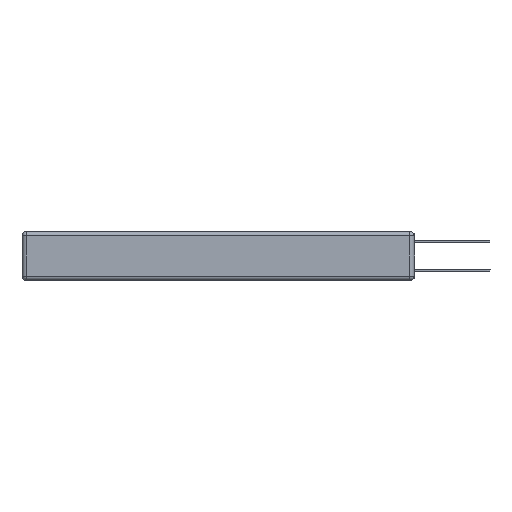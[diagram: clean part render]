
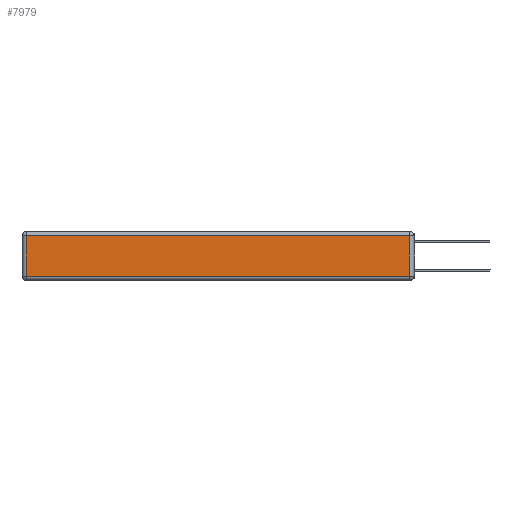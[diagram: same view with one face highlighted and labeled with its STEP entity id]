
A CAD part, left-side view. The second image highlights one B-rep face of the part: STEP entity #7979.
In plain terms, the highlighted planar face has unit normal (-1, 0, 0).
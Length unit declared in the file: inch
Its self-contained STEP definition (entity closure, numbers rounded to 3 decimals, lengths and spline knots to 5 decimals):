
#330 = VECTOR ( 'NONE', #3692, 39.37008 ) ;
#1174 = CARTESIAN_POINT ( 'NONE',  ( 0., 2.72, -0.343 ) ) ;
#1606 = ORIENTED_EDGE ( 'NONE', *, *, #9624, .T. ) ;
#1670 = VERTEX_POINT ( 'NONE', #16334 ) ;
#1967 = CARTESIAN_POINT ( 'NONE',  ( 0., 2.75, -0.03 ) ) ;
#2464 = EDGE_CURVE ( 'NONE', #16041, #1670, #11679, .T. ) ;
#2591 = DIRECTION ( 'NONE',  ( 0., 0., 1. ) ) ;
#3074 = CARTESIAN_POINT ( 'NONE',  ( 0., 0., -0.343 ) ) ;
#3692 = DIRECTION ( 'NONE',  ( 0., 0., -1. ) ) ;
#3740 = CARTESIAN_POINT ( 'NONE',  ( 0., 0.03, -0.313 ) ) ;
#4265 = LINE ( 'NONE', #9341, #16293 ) ;
#4415 = PLANE ( 'NONE',  #5699 ) ;
#5323 = VECTOR ( 'NONE', #11095, 39.37008 ) ;
#5699 = AXIS2_PLACEMENT_3D ( 'NONE', #3074, #6194, #8405 ) ;
#6194 = DIRECTION ( 'NONE',  ( -1., 0., 0. ) ) ;
#6601 = FACE_OUTER_BOUND ( 'NONE', #9531, .T. ) ;
#6953 = LINE ( 'NONE', #8497, #5323 ) ;
#7979 = ADVANCED_FACE ( 'NONE', ( #6601 ), #4415, .T. ) ;
#8330 = CARTESIAN_POINT ( 'NONE',  ( 0., 2.72, -0.03 ) ) ;
#8405 = DIRECTION ( 'NONE',  ( 0., 0., 1. ) ) ;
#8497 = CARTESIAN_POINT ( 'NONE',  ( 0., 0., -0.313 ) ) ;
#9250 = EDGE_CURVE ( 'NONE', #1670, #14311, #6953, .T. ) ;
#9341 = CARTESIAN_POINT ( 'NONE',  ( 0., 0.03, -0.343 ) ) ;
#9531 = EDGE_LOOP ( 'NONE', ( #9869, #1606, #12009, #12300 ) ) ;
#9624 = EDGE_CURVE ( 'NONE', #14311, #12112, #4265, .T. ) ;
#9869 = ORIENTED_EDGE ( 'NONE', *, *, #9250, .T. ) ;
#11095 = DIRECTION ( 'NONE',  ( 0., -1., 0. ) ) ;
#11517 = LINE ( 'NONE', #1967, #16929 ) ;
#11679 = LINE ( 'NONE', #1174, #330 ) ;
#12009 = ORIENTED_EDGE ( 'NONE', *, *, #14006, .T. ) ;
#12112 = VERTEX_POINT ( 'NONE', #12214 ) ;
#12214 = CARTESIAN_POINT ( 'NONE',  ( 0., 0.03, -0.03 ) ) ;
#12300 = ORIENTED_EDGE ( 'NONE', *, *, #2464, .T. ) ;
#14006 = EDGE_CURVE ( 'NONE', #12112, #16041, #11517, .T. ) ;
#14311 = VERTEX_POINT ( 'NONE', #3740 ) ;
#15248 = DIRECTION ( 'NONE',  ( 0., 1., 0. ) ) ;
#16041 = VERTEX_POINT ( 'NONE', #8330 ) ;
#16293 = VECTOR ( 'NONE', #2591, 39.37008 ) ;
#16334 = CARTESIAN_POINT ( 'NONE',  ( 0., 2.72, -0.313 ) ) ;
#16929 = VECTOR ( 'NONE', #15248, 39.37008 ) ;
